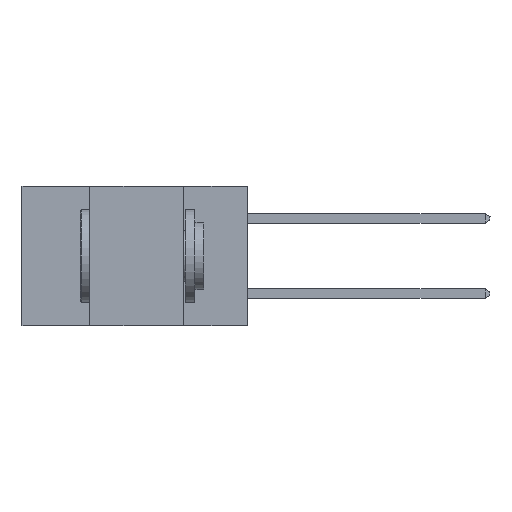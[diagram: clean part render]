
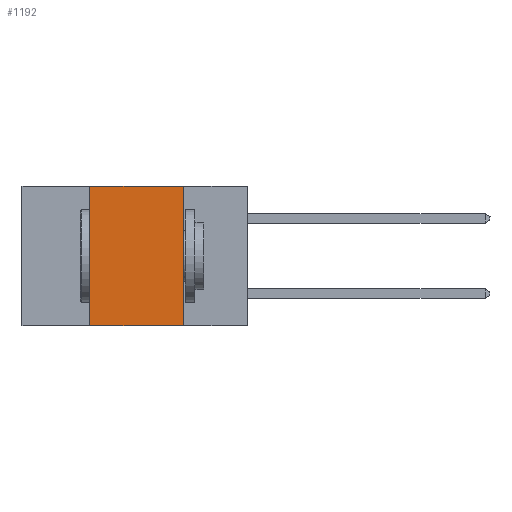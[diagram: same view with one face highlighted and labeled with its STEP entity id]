
A CAD part, left-side view. The second image highlights one B-rep face of the part: STEP entity #1192.
In plain terms, the highlighted planar face has unit normal (-1, 0, 0).
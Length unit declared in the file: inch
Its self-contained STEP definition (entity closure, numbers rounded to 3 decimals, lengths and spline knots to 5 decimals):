
#1192 = ADVANCED_FACE ( 'NONE', ( #13103 ), #19472, .F. ) ;
#1293 = ORIENTED_EDGE ( 'NONE', *, *, #7837, .F. ) ;
#3247 = EDGE_LOOP ( 'NONE', ( #1293, #6838, #10918, #23916 ) ) ;
#4194 = LINE ( 'NONE', #10038, #10736 ) ;
#4613 = AXIS2_PLACEMENT_3D ( 'NONE', #9167, #24408, #20205 ) ;
#6019 = CARTESIAN_POINT ( 'NONE',  ( 0., 0.17, 0. ) ) ;
#6838 = ORIENTED_EDGE ( 'NONE', *, *, #9263, .F. ) ;
#7299 = VERTEX_POINT ( 'NONE', #18358 ) ;
#7837 = EDGE_CURVE ( 'NONE', #11462, #7299, #17063, .T. ) ;
#7971 = LINE ( 'NONE', #18461, #19581 ) ;
#9167 = CARTESIAN_POINT ( 'NONE',  ( 0., 0.6, 0. ) ) ;
#9263 = EDGE_CURVE ( 'NONE', #10665, #11462, #20455, .T. ) ;
#9913 = VERTEX_POINT ( 'NONE', #20438 ) ;
#10038 = CARTESIAN_POINT ( 'NONE',  ( 0., 0.6, -0.37 ) ) ;
#10254 = VECTOR ( 'NONE', #25286, 39.37008 ) ;
#10665 = VERTEX_POINT ( 'NONE', #10881 ) ;
#10736 = VECTOR ( 'NONE', #18191, 39.37008 ) ;
#10881 = CARTESIAN_POINT ( 'NONE',  ( 0., 0.42, 0. ) ) ;
#10918 = ORIENTED_EDGE ( 'NONE', *, *, #26569, .F. ) ;
#11388 = VECTOR ( 'NONE', #12064, 39.37008 ) ;
#11462 = VERTEX_POINT ( 'NONE', #25902 ) ;
#12064 = DIRECTION ( 'NONE',  ( 0., -1., 0. ) ) ;
#13103 = FACE_OUTER_BOUND ( 'NONE', #3247, .T. ) ;
#16068 = CARTESIAN_POINT ( 'NONE',  ( 0., 0.6, 0. ) ) ;
#17063 = LINE ( 'NONE', #6019, #10254 ) ;
#18191 = DIRECTION ( 'NONE',  ( 0., -1., 0. ) ) ;
#18358 = CARTESIAN_POINT ( 'NONE',  ( 0., 0.17, -0.37 ) ) ;
#18461 = CARTESIAN_POINT ( 'NONE',  ( 0., 0.42, 0. ) ) ;
#19472 = PLANE ( 'NONE',  #4613 ) ;
#19581 = VECTOR ( 'NONE', #26574, 39.37008 ) ;
#20205 = DIRECTION ( 'NONE',  ( 0., 0., -1. ) ) ;
#20438 = CARTESIAN_POINT ( 'NONE',  ( 0., 0.42, -0.37 ) ) ;
#20455 = LINE ( 'NONE', #16068, #11388 ) ;
#22681 = EDGE_CURVE ( 'NONE', #9913, #7299, #4194, .T. ) ;
#23916 = ORIENTED_EDGE ( 'NONE', *, *, #22681, .T. ) ;
#24408 = DIRECTION ( 'NONE',  ( 1., 0., 0. ) ) ;
#25286 = DIRECTION ( 'NONE',  ( 0., 0., -1. ) ) ;
#25902 = CARTESIAN_POINT ( 'NONE',  ( 0., 0.17, 0. ) ) ;
#26569 = EDGE_CURVE ( 'NONE', #9913, #10665, #7971, .T. ) ;
#26574 = DIRECTION ( 'NONE',  ( 0., 0., 1. ) ) ;
